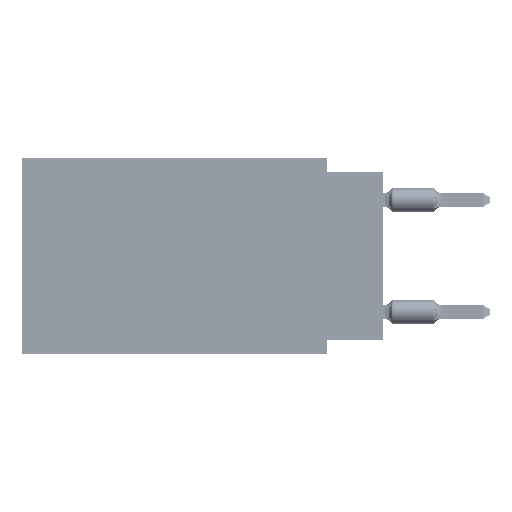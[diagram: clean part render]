
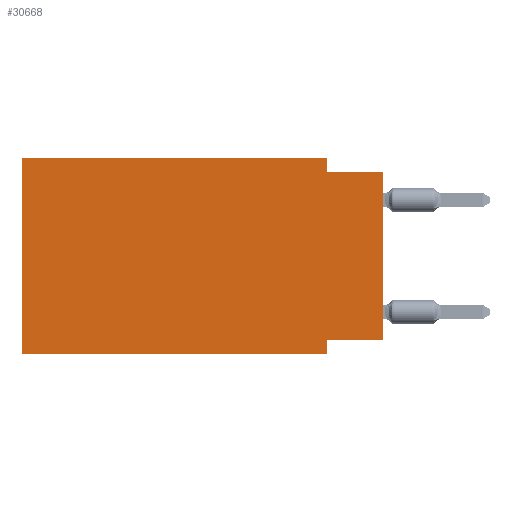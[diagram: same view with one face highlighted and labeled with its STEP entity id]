
A CAD part, left-side view. The second image highlights one B-rep face of the part: STEP entity #30668.
In plain terms, the highlighted planar face has unit normal (-1, 0, 0).
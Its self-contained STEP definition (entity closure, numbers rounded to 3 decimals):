
#127 = EDGE_CURVE ( 'NONE', #72251, #101264, #24438, .T. ) ;
#2574 = LINE ( 'NONE', #81614, #77790 ) ;
#3880 = EDGE_CURVE ( 'NONE', #56021, #35232, #2574, .T. ) ;
#10122 = VERTEX_POINT ( 'NONE', #66976 ) ;
#12457 = DIRECTION ( 'NONE',  ( 0., -1., 0. ) ) ;
#12685 = AXIS2_PLACEMENT_3D ( 'NONE', #73611, #29269, #106102 ) ;
#14848 = ORIENTED_EDGE ( 'NONE', *, *, #68274, .F. ) ;
#16473 = CARTESIAN_POINT ( 'NONE',  ( 0., 0., 0. ) ) ;
#20271 = ORIENTED_EDGE ( 'NONE', *, *, #36636, .T. ) ;
#22990 = EDGE_CURVE ( 'NONE', #93049, #75466, #84538, .T. ) ;
#24438 = LINE ( 'NONE', #16473, #104029 ) ;
#26786 = ORIENTED_EDGE ( 'NONE', *, *, #104486, .F. ) ;
#29269 = DIRECTION ( 'NONE',  ( 1., 0., 0. ) ) ;
#30142 = ORIENTED_EDGE ( 'NONE', *, *, #87692, .F. ) ;
#30390 = ORIENTED_EDGE ( 'NONE', *, *, #101935, .F. ) ;
#30648 = LINE ( 'NONE', #101190, #90794 ) ;
#30668 = ADVANCED_FACE ( 'NONE', ( #71386 ), #45769, .F. ) ;
#35232 = VERTEX_POINT ( 'NONE', #80113 ) ;
#36636 = EDGE_CURVE ( 'NONE', #56021, #75466, #110230, .T. ) ;
#37280 = DIRECTION ( 'NONE',  ( 0., 0., 1. ) ) ;
#37866 = ORIENTED_EDGE ( 'NONE', *, *, #3880, .F. ) ;
#41685 = CARTESIAN_POINT ( 'NONE',  ( 0., 0., -8.255 ) ) ;
#45589 = VECTOR ( 'NONE', #46096, 1000. ) ;
#45769 = PLANE ( 'NONE',  #12685 ) ;
#46096 = DIRECTION ( 'NONE',  ( 0., 0., -1. ) ) ;
#46115 = VECTOR ( 'NONE', #59893, 1000. ) ;
#49146 = DIRECTION ( 'NONE',  ( 0., -1., 0. ) ) ;
#49337 = DIRECTION ( 'NONE',  ( 0., -1., 0. ) ) ;
#51909 = CARTESIAN_POINT ( 'NONE',  ( 0., 2.54, -8.255 ) ) ;
#52445 = VERTEX_POINT ( 'NONE', #96335 ) ;
#56021 = VERTEX_POINT ( 'NONE', #94495 ) ;
#57987 = VECTOR ( 'NONE', #49146, 1000. ) ;
#58361 = CARTESIAN_POINT ( 'NONE',  ( 0., 2.54, -8.89 ) ) ;
#59893 = DIRECTION ( 'NONE',  ( 0., 1., 0. ) ) ;
#60846 = VECTOR ( 'NONE', #109597, 1000. ) ;
#66976 = CARTESIAN_POINT ( 'NONE',  ( 0., 2.54, -0.635 ) ) ;
#68274 = EDGE_CURVE ( 'NONE', #10122, #101264, #30648, .T. ) ;
#71386 = FACE_OUTER_BOUND ( 'NONE', #107380, .T. ) ;
#72251 = VERTEX_POINT ( 'NONE', #91290 ) ;
#73611 = CARTESIAN_POINT ( 'NONE',  ( 0., 16.383, 0. ) ) ;
#74941 = CARTESIAN_POINT ( 'NONE',  ( 0., 16.383, -8.89 ) ) ;
#75466 = VERTEX_POINT ( 'NONE', #110327 ) ;
#75751 = CARTESIAN_POINT ( 'NONE',  ( 0., 0., -0.635 ) ) ;
#77790 = VECTOR ( 'NONE', #37280, 1000. ) ;
#80113 = CARTESIAN_POINT ( 'NONE',  ( 0., 16.383, 0. ) ) ;
#81614 = CARTESIAN_POINT ( 'NONE',  ( 0., 16.383, 0. ) ) ;
#84538 = LINE ( 'NONE', #58361, #60846 ) ;
#85547 = ORIENTED_EDGE ( 'NONE', *, *, #127, .T. ) ;
#85917 = VECTOR ( 'NONE', #49337, 1000. ) ;
#87692 = EDGE_CURVE ( 'NONE', #72251, #93049, #92361, .T. ) ;
#90794 = VECTOR ( 'NONE', #12457, 1000. ) ;
#91290 = CARTESIAN_POINT ( 'NONE',  ( 0., 0., -8.255 ) ) ;
#92160 = LINE ( 'NONE', #107543, #45589 ) ;
#92361 = LINE ( 'NONE', #41685, #46115 ) ;
#92364 = ORIENTED_EDGE ( 'NONE', *, *, #22990, .F. ) ;
#92400 = CARTESIAN_POINT ( 'NONE',  ( 0., 16.383, 0. ) ) ;
#93049 = VERTEX_POINT ( 'NONE', #51909 ) ;
#94495 = CARTESIAN_POINT ( 'NONE',  ( 0., 16.383, -8.89 ) ) ;
#95549 = DIRECTION ( 'NONE',  ( 0., 0., 1. ) ) ;
#96335 = CARTESIAN_POINT ( 'NONE',  ( 0., 2.54, 0. ) ) ;
#101190 = CARTESIAN_POINT ( 'NONE',  ( 0., 0., -0.635 ) ) ;
#101264 = VERTEX_POINT ( 'NONE', #75751 ) ;
#101935 = EDGE_CURVE ( 'NONE', #35232, #52445, #110587, .T. ) ;
#104029 = VECTOR ( 'NONE', #95549, 1000. ) ;
#104486 = EDGE_CURVE ( 'NONE', #52445, #10122, #92160, .T. ) ;
#106102 = DIRECTION ( 'NONE',  ( 0., 0., -1. ) ) ;
#107380 = EDGE_LOOP ( 'NONE', ( #85547, #14848, #26786, #30390, #37866, #20271, #92364, #30142 ) ) ;
#107543 = CARTESIAN_POINT ( 'NONE',  ( 0., 2.54, 0. ) ) ;
#109597 = DIRECTION ( 'NONE',  ( 0., 0., -1. ) ) ;
#110230 = LINE ( 'NONE', #74941, #85917 ) ;
#110327 = CARTESIAN_POINT ( 'NONE',  ( 0., 2.54, -8.89 ) ) ;
#110587 = LINE ( 'NONE', #92400, #57987 ) ;
